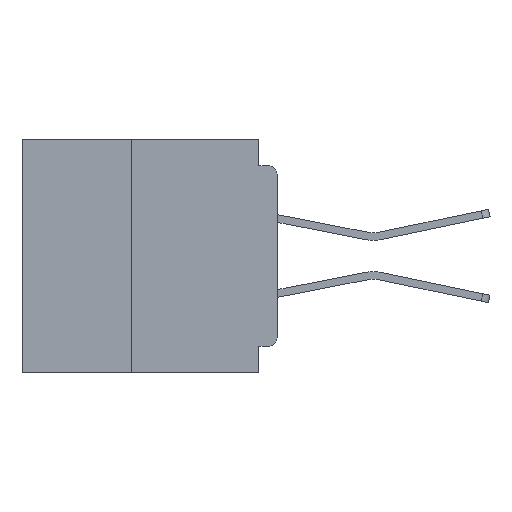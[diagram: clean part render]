
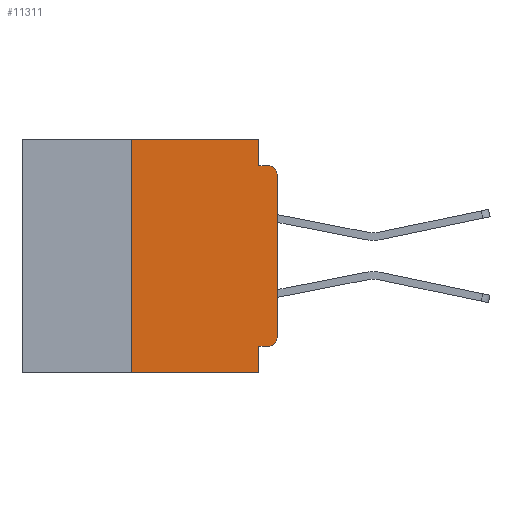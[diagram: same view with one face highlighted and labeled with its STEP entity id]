
A CAD part, left-side view. The second image highlights one B-rep face of the part: STEP entity #11311.
In plain terms, the highlighted planar face has unit normal (-1, 0, 0).
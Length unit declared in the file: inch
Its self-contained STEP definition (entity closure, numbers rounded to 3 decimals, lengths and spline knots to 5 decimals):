
#52 = CARTESIAN_POINT ( 'NONE',  ( 0., 0.031, -0.045 ) ) ;
#765 = ORIENTED_EDGE ( 'NONE', *, *, #33628, .F. ) ;
#1302 = CARTESIAN_POINT ( 'NONE',  ( 0., 0.015, -0.355 ) ) ;
#1460 = VECTOR ( 'NONE', #16078, 39.37008 ) ;
#1622 = DIRECTION ( 'NONE',  ( 0., 0., 1. ) ) ;
#3325 = CARTESIAN_POINT ( 'NONE',  ( 0., 0.437, 0. ) ) ;
#3424 = VERTEX_POINT ( 'NONE', #32660 ) ;
#3471 = ORIENTED_EDGE ( 'NONE', *, *, #20917, .T. ) ;
#4284 = VERTEX_POINT ( 'NONE', #20367 ) ;
#4711 = CARTESIAN_POINT ( 'NONE',  ( 0., 0.437, -0.4 ) ) ;
#4812 = DIRECTION ( 'NONE',  ( -1., 0., 0. ) ) ;
#5856 = LINE ( 'NONE', #21147, #20238 ) ;
#5877 = CARTESIAN_POINT ( 'NONE',  ( 0., 0.031, -0.4 ) ) ;
#7078 = CARTESIAN_POINT ( 'NONE',  ( 0., 0.015, -0.06 ) ) ;
#7609 = VERTEX_POINT ( 'NONE', #5877 ) ;
#9411 = CARTESIAN_POINT ( 'NONE',  ( 0., 0.031, 0. ) ) ;
#9834 = AXIS2_PLACEMENT_3D ( 'NONE', #7078, #27056, #9971 ) ;
#9971 = DIRECTION ( 'NONE',  ( 0., 0., -1. ) ) ;
#10019 = LINE ( 'NONE', #11813, #31829 ) ;
#10356 = CARTESIAN_POINT ( 'NONE',  ( 0., 0.25, -0.4 ) ) ;
#11311 = ADVANCED_FACE ( 'NONE', ( #14284 ), #34650, .F. ) ;
#11813 = CARTESIAN_POINT ( 'NONE',  ( 0., 0., -0.045 ) ) ;
#11863 = LINE ( 'NONE', #18380, #20384 ) ;
#12006 = VECTOR ( 'NONE', #14040, 39.37008 ) ;
#12048 = DIRECTION ( 'NONE',  ( 0., 0., -1. ) ) ;
#12495 = EDGE_LOOP ( 'NONE', ( #14407, #3471, #19428, #31059, #22911, #765, #14186, #31788, #36359, #25134 ) ) ;
#12834 = VECTOR ( 'NONE', #1622, 39.37008 ) ;
#12934 = VERTEX_POINT ( 'NONE', #24915 ) ;
#13923 = EDGE_CURVE ( 'NONE', #24491, #27379, #29707, .T. ) ;
#14040 = DIRECTION ( 'NONE',  ( 0., 0., 1. ) ) ;
#14186 = ORIENTED_EDGE ( 'NONE', *, *, #26817, .T. ) ;
#14284 = FACE_OUTER_BOUND ( 'NONE', #12495, .T. ) ;
#14407 = ORIENTED_EDGE ( 'NONE', *, *, #28017, .T. ) ;
#14419 = EDGE_CURVE ( 'NONE', #24491, #4284, #11863, .T. ) ;
#14931 = EDGE_CURVE ( 'NONE', #35130, #21409, #10019, .T. ) ;
#15045 = EDGE_CURVE ( 'NONE', #3424, #35130, #27398, .T. ) ;
#15082 = CARTESIAN_POINT ( 'NONE',  ( 0., 0.015, -0.045 ) ) ;
#15407 = DIRECTION ( 'NONE',  ( 0., -1., 0. ) ) ;
#15651 = LINE ( 'NONE', #4711, #29840 ) ;
#15725 = EDGE_CURVE ( 'NONE', #27869, #3424, #5856, .T. ) ;
#16078 = DIRECTION ( 'NONE',  ( 0., 0., -1. ) ) ;
#16818 = LINE ( 'NONE', #33047, #1460 ) ;
#18022 = AXIS2_PLACEMENT_3D ( 'NONE', #3325, #29076, #12048 ) ;
#18380 = CARTESIAN_POINT ( 'NONE',  ( 0., 0., -0.355 ) ) ;
#18887 = VERTEX_POINT ( 'NONE', #28771 ) ;
#19428 = ORIENTED_EDGE ( 'NONE', *, *, #14931, .F. ) ;
#20238 = VECTOR ( 'NONE', #15407, 39.37008 ) ;
#20367 = CARTESIAN_POINT ( 'NONE',  ( 0., 0.031, -0.355 ) ) ;
#20384 = VECTOR ( 'NONE', #35328, 39.37008 ) ;
#20917 = EDGE_CURVE ( 'NONE', #12934, #21409, #23399, .T. ) ;
#21147 = CARTESIAN_POINT ( 'NONE',  ( 0., 0.437, 0. ) ) ;
#21409 = VERTEX_POINT ( 'NONE', #15082 ) ;
#22002 = CARTESIAN_POINT ( 'NONE',  ( 0., 0.015, -0.34 ) ) ;
#22063 = CARTESIAN_POINT ( 'NONE',  ( 0., 0.25, 0. ) ) ;
#22144 = DIRECTION ( 'NONE',  ( 0., -1., 0. ) ) ;
#22911 = ORIENTED_EDGE ( 'NONE', *, *, #15725, .F. ) ;
#23209 = EDGE_CURVE ( 'NONE', #4284, #7609, #16818, .T. ) ;
#23399 = CIRCLE ( 'NONE', #9834, 0.015 ) ;
#24289 = AXIS2_PLACEMENT_3D ( 'NONE', #22002, #4812, #24851 ) ;
#24491 = VERTEX_POINT ( 'NONE', #1302 ) ;
#24851 = DIRECTION ( 'NONE',  ( 0., 0., -1. ) ) ;
#24915 = CARTESIAN_POINT ( 'NONE',  ( 0., 0., -0.06 ) ) ;
#25134 = ORIENTED_EDGE ( 'NONE', *, *, #13923, .T. ) ;
#26817 = EDGE_CURVE ( 'NONE', #18887, #7609, #15651, .T. ) ;
#27056 = DIRECTION ( 'NONE',  ( -1., 0., 0. ) ) ;
#27379 = VERTEX_POINT ( 'NONE', #30847 ) ;
#27398 = LINE ( 'NONE', #9411, #34930 ) ;
#27869 = VERTEX_POINT ( 'NONE', #22063 ) ;
#28017 = EDGE_CURVE ( 'NONE', #27379, #12934, #34678, .T. ) ;
#28203 = CARTESIAN_POINT ( 'NONE',  ( 0., 0., 0. ) ) ;
#28771 = CARTESIAN_POINT ( 'NONE',  ( 0., 0.25, -0.4 ) ) ;
#28845 = LINE ( 'NONE', #10356, #12834 ) ;
#29076 = DIRECTION ( 'NONE',  ( 1., 0., 0. ) ) ;
#29707 = CIRCLE ( 'NONE', #24289, 0.015 ) ;
#29840 = VECTOR ( 'NONE', #22144, 39.37008 ) ;
#30847 = CARTESIAN_POINT ( 'NONE',  ( 0., 0., -0.34 ) ) ;
#31059 = ORIENTED_EDGE ( 'NONE', *, *, #15045, .F. ) ;
#31788 = ORIENTED_EDGE ( 'NONE', *, *, #23209, .F. ) ;
#31829 = VECTOR ( 'NONE', #34417, 39.37008 ) ;
#32195 = DIRECTION ( 'NONE',  ( 0., 0., -1. ) ) ;
#32660 = CARTESIAN_POINT ( 'NONE',  ( 0., 0.031, 0. ) ) ;
#33047 = CARTESIAN_POINT ( 'NONE',  ( 0., 0.031, -0.4 ) ) ;
#33628 = EDGE_CURVE ( 'NONE', #18887, #27869, #28845, .T. ) ;
#34417 = DIRECTION ( 'NONE',  ( 0., -1., 0. ) ) ;
#34650 = PLANE ( 'NONE',  #18022 ) ;
#34678 = LINE ( 'NONE', #28203, #12006 ) ;
#34930 = VECTOR ( 'NONE', #32195, 39.37008 ) ;
#35130 = VERTEX_POINT ( 'NONE', #52 ) ;
#35328 = DIRECTION ( 'NONE',  ( 0., 1., 0. ) ) ;
#36359 = ORIENTED_EDGE ( 'NONE', *, *, #14419, .F. ) ;
